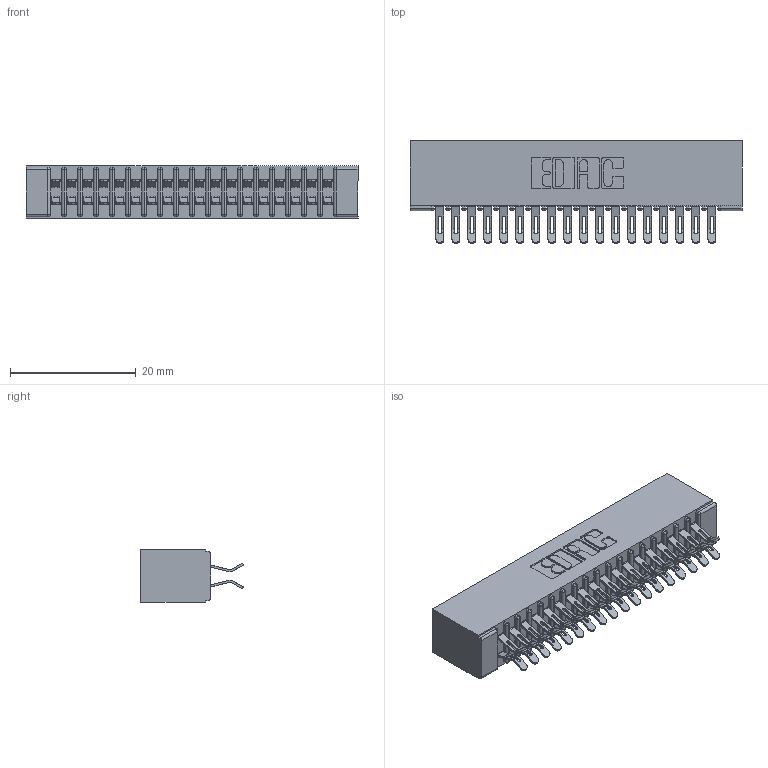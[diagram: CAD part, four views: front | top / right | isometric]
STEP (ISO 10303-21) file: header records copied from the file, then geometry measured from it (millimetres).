
FILE_DESCRIPTION (( 'STEP AP203' ), '1' );
FILE_NAME ('391-036-555-201.STEP', '2018-08-08T23:36:55', ( '' ), ( '' ), 'SwSTEP 2.0', 'SolidWorks 2016', '' );
FILE_SCHEMA (( 'CONFIG_CONTROL_DESIGN' ));
Length unit declared in the file: inch
Products named in the file (3): 341 Part_No Mounting Lugs; 341-292-001_341-292-155; 391-036-555-201
Assembly tree (37 placements, depth 2):
  391-036-555-201
    341 Part_No Mounting Lugs
    341-292-001_341-292-155  x36
Bounding box: 52.7 x 16.31 x 8.38 mm (x, y, z)
Volume: 3186 mm3; surface area: 7345.4 mm2
Topology: 37 solids, 37 shells, 2916 faces, 8698 edges, 5662 vertices
Faces by surface type: plane 1576, cylinder 1268, sphere 38, torus 34
Entity records: 25173 total; most frequent: CARTESIAN_POINT 4200, ORIENTED_EDGE 4160, DIRECTION 4082, EDGE_CURVE 2080, LINE 1642, VECTOR 1642, VERTEX_POINT 1322, AXIS2_PLACEMENT_3D 1220
